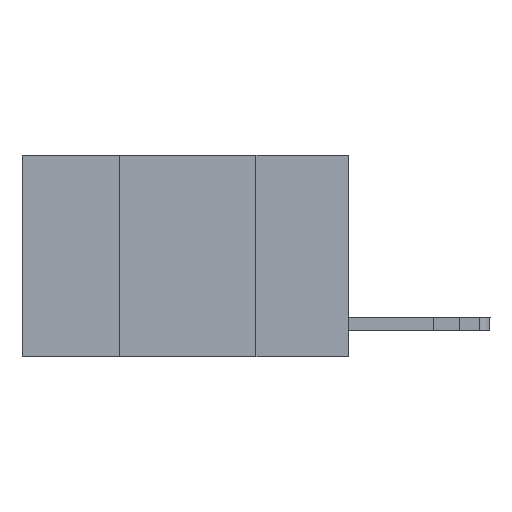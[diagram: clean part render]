
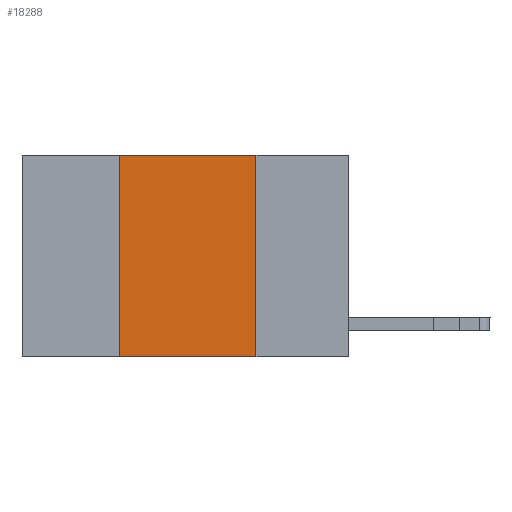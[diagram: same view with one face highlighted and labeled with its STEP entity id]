
A CAD part, left-side view. The second image highlights one B-rep face of the part: STEP entity #18288.
In plain terms, the highlighted planar face has unit normal (-1, 0, 0).
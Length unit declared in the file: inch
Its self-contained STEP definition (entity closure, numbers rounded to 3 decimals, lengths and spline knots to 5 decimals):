
#418 = DIRECTION ( 'NONE',  ( 0., 0., -1. ) ) ;
#1937 = LINE ( 'NONE', #3438, #5014 ) ;
#2617 = DIRECTION ( 'NONE',  ( 0., -1., 0. ) ) ;
#2728 = VECTOR ( 'NONE', #14864, 39.37008 ) ;
#3367 = DIRECTION ( 'NONE',  ( 1., 0., 0. ) ) ;
#3438 = CARTESIAN_POINT ( 'NONE',  ( 0., 0.17, 0. ) ) ;
#5014 = VECTOR ( 'NONE', #418, 39.37008 ) ;
#5051 = CARTESIAN_POINT ( 'NONE',  ( 0., 0.42, 0. ) ) ;
#6740 = ORIENTED_EDGE ( 'NONE', *, *, #10691, .F. ) ;
#7249 = LINE ( 'NONE', #16279, #14530 ) ;
#7453 = ORIENTED_EDGE ( 'NONE', *, *, #12389, .T. ) ;
#7758 = ORIENTED_EDGE ( 'NONE', *, *, #13132, .F. ) ;
#7804 = DIRECTION ( 'NONE',  ( 0., 0., -1. ) ) ;
#7832 = EDGE_LOOP ( 'NONE', ( #7758, #6740, #11040, #7453 ) ) ;
#7903 = CARTESIAN_POINT ( 'NONE',  ( 0., 0.17, 0. ) ) ;
#9302 = FACE_OUTER_BOUND ( 'NONE', #7832, .T. ) ;
#10691 = EDGE_CURVE ( 'NONE', #17439, #12557, #7249, .T. ) ;
#11040 = ORIENTED_EDGE ( 'NONE', *, *, #14169, .F. ) ;
#11386 = DIRECTION ( 'NONE',  ( 0., 0., 1. ) ) ;
#12389 = EDGE_CURVE ( 'NONE', #15936, #13107, #16249, .T. ) ;
#12557 = VERTEX_POINT ( 'NONE', #7903 ) ;
#13107 = VERTEX_POINT ( 'NONE', #18121 ) ;
#13132 = EDGE_CURVE ( 'NONE', #12557, #13107, #1937, .T. ) ;
#14169 = EDGE_CURVE ( 'NONE', #15936, #17439, #16059, .T. ) ;
#14530 = VECTOR ( 'NONE', #2617, 39.37008 ) ;
#14864 = DIRECTION ( 'NONE',  ( 0., -1., 0. ) ) ;
#14917 = VECTOR ( 'NONE', #11386, 39.37008 ) ;
#15356 = AXIS2_PLACEMENT_3D ( 'NONE', #15555, #3367, #7804 ) ;
#15555 = CARTESIAN_POINT ( 'NONE',  ( 0., 0.6, 0. ) ) ;
#15936 = VERTEX_POINT ( 'NONE', #18993 ) ;
#16059 = LINE ( 'NONE', #19350, #14917 ) ;
#16249 = LINE ( 'NONE', #19649, #2728 ) ;
#16279 = CARTESIAN_POINT ( 'NONE',  ( 0., 0.6, 0. ) ) ;
#17238 = PLANE ( 'NONE',  #15356 ) ;
#17439 = VERTEX_POINT ( 'NONE', #5051 ) ;
#18121 = CARTESIAN_POINT ( 'NONE',  ( 0., 0.17, -0.37 ) ) ;
#18288 = ADVANCED_FACE ( 'NONE', ( #9302 ), #17238, .F. ) ;
#18993 = CARTESIAN_POINT ( 'NONE',  ( 0., 0.42, -0.37 ) ) ;
#19350 = CARTESIAN_POINT ( 'NONE',  ( 0., 0.42, 0. ) ) ;
#19649 = CARTESIAN_POINT ( 'NONE',  ( 0., 0.6, -0.37 ) ) ;
